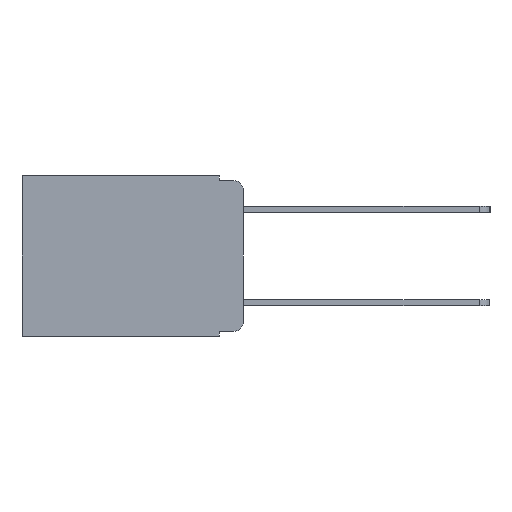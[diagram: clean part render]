
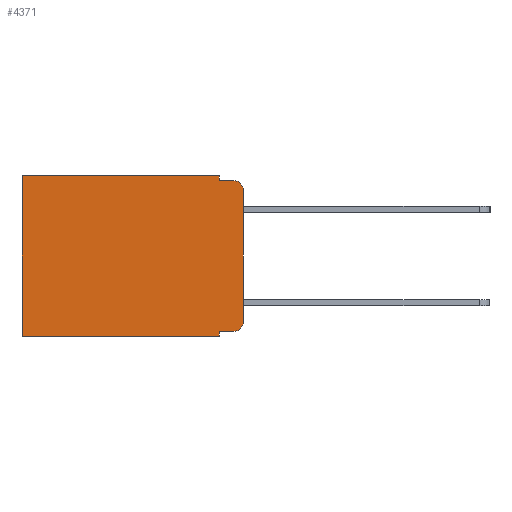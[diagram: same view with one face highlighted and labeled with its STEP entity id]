
A CAD part, left-side view. The second image highlights one B-rep face of the part: STEP entity #4371.
In plain terms, the highlighted planar face has unit normal (-1, 0, 0).
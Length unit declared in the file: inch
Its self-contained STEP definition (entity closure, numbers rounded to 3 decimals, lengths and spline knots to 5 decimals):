
#30 = AXIS2_PLACEMENT_3D ( 'NONE', #2726, #11863, #15353 ) ;
#502 = ORIENTED_EDGE ( 'NONE', *, *, #15803, .F. ) ;
#997 = ORIENTED_EDGE ( 'NONE', *, *, #14239, .T. ) ;
#1011 = LINE ( 'NONE', #1263, #7807 ) ;
#1263 = CARTESIAN_POINT ( 'NONE',  ( 0.298, 0.051, 0. ) ) ;
#1337 = CARTESIAN_POINT ( 'NONE',  ( 0.298, 0.051, -0.343 ) ) ;
#1488 = ORIENTED_EDGE ( 'NONE', *, *, #13465, .F. ) ;
#1731 = AXIS2_PLACEMENT_3D ( 'NONE', #11121, #3268, #12266 ) ;
#2386 = VERTEX_POINT ( 'NONE', #3601 ) ;
#2558 = LINE ( 'NONE', #6052, #9407 ) ;
#2726 = CARTESIAN_POINT ( 'NONE',  ( 0.298, 0., 0. ) ) ;
#3268 = DIRECTION ( 'NONE',  ( -1., 0., 0. ) ) ;
#3538 = VECTOR ( 'NONE', #16137, 39.37008 ) ;
#3601 = CARTESIAN_POINT ( 'NONE',  ( 0.298, 0., -0.313 ) ) ;
#3665 = CARTESIAN_POINT ( 'NONE',  ( 0.298, 0.051, -0.01 ) ) ;
#3813 = CARTESIAN_POINT ( 'NONE',  ( 0.298, 0.02, -0.01 ) ) ;
#4371 = ADVANCED_FACE ( 'NONE', ( #8188 ), #9573, .F. ) ;
#4409 = VERTEX_POINT ( 'NONE', #14012 ) ;
#4485 = CARTESIAN_POINT ( 'NONE',  ( 0.298, 0., -0.343 ) ) ;
#4816 = VECTOR ( 'NONE', #12047, 39.37008 ) ;
#4833 = CARTESIAN_POINT ( 'NONE',  ( 0.298, 0.473, 0. ) ) ;
#5301 = DIRECTION ( 'NONE',  ( 0., 0., -1. ) ) ;
#5589 = VERTEX_POINT ( 'NONE', #11667 ) ;
#5932 = ORIENTED_EDGE ( 'NONE', *, *, #10419, .T. ) ;
#5968 = EDGE_LOOP ( 'NONE', ( #502, #997, #1488, #8584, #8961, #5932, #9340, #6374, #6808, #13107 ) ) ;
#6052 = CARTESIAN_POINT ( 'NONE',  ( 0.298, 0.051, -0.333 ) ) ;
#6163 = CARTESIAN_POINT ( 'NONE',  ( 0.298, 0.051, -0.01 ) ) ;
#6374 = ORIENTED_EDGE ( 'NONE', *, *, #9634, .F. ) ;
#6375 = VERTEX_POINT ( 'NONE', #4833 ) ;
#6808 = ORIENTED_EDGE ( 'NONE', *, *, #8022, .T. ) ;
#6877 = CARTESIAN_POINT ( 'NONE',  ( 0.298, 0.051, 0. ) ) ;
#7037 = DIRECTION ( 'NONE',  ( -1., 0., 0. ) ) ;
#7148 = EDGE_CURVE ( 'NONE', #4409, #2386, #7271, .T. ) ;
#7271 = CIRCLE ( 'NONE', #15615, 0.02 ) ;
#7412 = DIRECTION ( 'NONE',  ( 0., -1., 0. ) ) ;
#7807 = VECTOR ( 'NONE', #11935, 39.37008 ) ;
#8002 = LINE ( 'NONE', #6163, #16545 ) ;
#8022 = EDGE_CURVE ( 'NONE', #10203, #4409, #2558, .T. ) ;
#8188 = FACE_OUTER_BOUND ( 'NONE', #5968, .T. ) ;
#8584 = ORIENTED_EDGE ( 'NONE', *, *, #11207, .F. ) ;
#8627 = VECTOR ( 'NONE', #11736, 39.37008 ) ;
#8961 = ORIENTED_EDGE ( 'NONE', *, *, #10838, .T. ) ;
#9340 = ORIENTED_EDGE ( 'NONE', *, *, #11408, .F. ) ;
#9407 = VECTOR ( 'NONE', #7412, 39.37008 ) ;
#9525 = LINE ( 'NONE', #4485, #15297 ) ;
#9573 = PLANE ( 'NONE',  #30 ) ;
#9634 = EDGE_CURVE ( 'NONE', #10203, #13960, #11762, .T. ) ;
#9674 = CIRCLE ( 'NONE', #1731, 0.02 ) ;
#9953 = DIRECTION ( 'NONE',  ( 0., -1., 0. ) ) ;
#10203 = VERTEX_POINT ( 'NONE', #15856 ) ;
#10419 = EDGE_CURVE ( 'NONE', #6375, #15456, #11380, .T. ) ;
#10838 = EDGE_CURVE ( 'NONE', #5589, #6375, #14200, .T. ) ;
#11041 = CARTESIAN_POINT ( 'NONE',  ( 0.298, 0.473, -0.343 ) ) ;
#11121 = CARTESIAN_POINT ( 'NONE',  ( 0.298, 0.02, -0.03 ) ) ;
#11207 = EDGE_CURVE ( 'NONE', #5589, #12803, #1011, .T. ) ;
#11380 = LINE ( 'NONE', #11567, #14383 ) ;
#11408 = EDGE_CURVE ( 'NONE', #13960, #15456, #9525, .T. ) ;
#11567 = CARTESIAN_POINT ( 'NONE',  ( 0.298, 0.473, 0. ) ) ;
#11667 = CARTESIAN_POINT ( 'NONE',  ( 0.298, 0.051, 0. ) ) ;
#11736 = DIRECTION ( 'NONE',  ( 0., 0., -1. ) ) ;
#11762 = LINE ( 'NONE', #6877, #8627 ) ;
#11863 = DIRECTION ( 'NONE',  ( 1., 0., 0. ) ) ;
#11935 = DIRECTION ( 'NONE',  ( 0., 0., -1. ) ) ;
#12047 = DIRECTION ( 'NONE',  ( 0., 1., 0. ) ) ;
#12266 = DIRECTION ( 'NONE',  ( 0., 0., -1. ) ) ;
#12648 = CARTESIAN_POINT ( 'NONE',  ( 0.298, 0., 0. ) ) ;
#12803 = VERTEX_POINT ( 'NONE', #3665 ) ;
#13107 = ORIENTED_EDGE ( 'NONE', *, *, #7148, .T. ) ;
#13465 = EDGE_CURVE ( 'NONE', #12803, #14667, #8002, .T. ) ;
#13570 = LINE ( 'NONE', #12648, #3538 ) ;
#13960 = VERTEX_POINT ( 'NONE', #1337 ) ;
#14012 = CARTESIAN_POINT ( 'NONE',  ( 0.298, 0.02, -0.333 ) ) ;
#14067 = CARTESIAN_POINT ( 'NONE',  ( 0.298, 0.02, -0.313 ) ) ;
#14200 = LINE ( 'NONE', #14310, #4816 ) ;
#14239 = EDGE_CURVE ( 'NONE', #14653, #14667, #9674, .T. ) ;
#14310 = CARTESIAN_POINT ( 'NONE',  ( 0.298, 0., 0. ) ) ;
#14383 = VECTOR ( 'NONE', #5301, 39.37008 ) ;
#14653 = VERTEX_POINT ( 'NONE', #16223 ) ;
#14667 = VERTEX_POINT ( 'NONE', #3813 ) ;
#15266 = DIRECTION ( 'NONE',  ( 0., 0., -1. ) ) ;
#15297 = VECTOR ( 'NONE', #16694, 39.37008 ) ;
#15353 = DIRECTION ( 'NONE',  ( 0., 0., -1. ) ) ;
#15456 = VERTEX_POINT ( 'NONE', #11041 ) ;
#15615 = AXIS2_PLACEMENT_3D ( 'NONE', #14067, #7037, #15266 ) ;
#15803 = EDGE_CURVE ( 'NONE', #14653, #2386, #13570, .T. ) ;
#15856 = CARTESIAN_POINT ( 'NONE',  ( 0.298, 0.051, -0.333 ) ) ;
#16137 = DIRECTION ( 'NONE',  ( 0., 0., -1. ) ) ;
#16223 = CARTESIAN_POINT ( 'NONE',  ( 0.298, 0., -0.03 ) ) ;
#16545 = VECTOR ( 'NONE', #9953, 39.37008 ) ;
#16694 = DIRECTION ( 'NONE',  ( 0., 1., 0. ) ) ;
